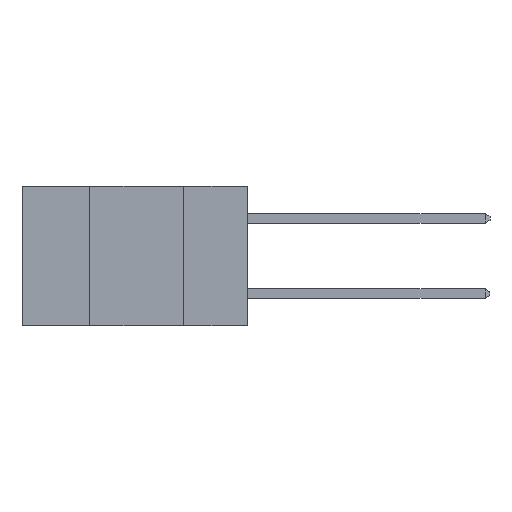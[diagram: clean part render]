
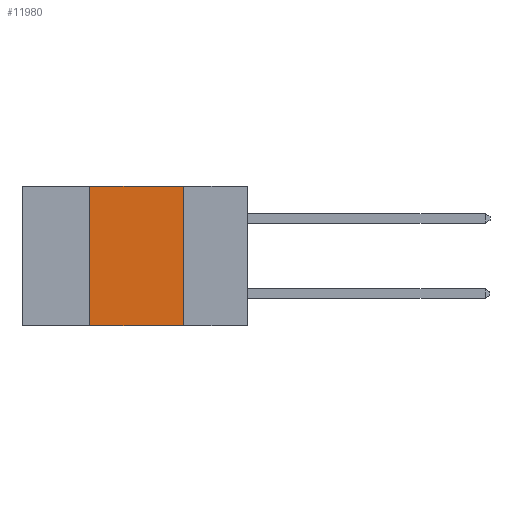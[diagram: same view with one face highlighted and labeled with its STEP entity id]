
A CAD part, left-side view. The second image highlights one B-rep face of the part: STEP entity #11980.
In plain terms, the highlighted planar face has unit normal (-1, 0, 0).
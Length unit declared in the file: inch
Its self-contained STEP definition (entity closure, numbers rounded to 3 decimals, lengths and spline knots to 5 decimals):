
#493 = VERTEX_POINT ( 'NONE', #1086 ) ;
#560 = VECTOR ( 'NONE', #1046, 39.37008 ) ;
#861 = ORIENTED_EDGE ( 'NONE', *, *, #2128, .F. ) ;
#951 = AXIS2_PLACEMENT_3D ( 'NONE', #5636, #13935, #6883 ) ;
#1046 = DIRECTION ( 'NONE',  ( 0., 0., -1. ) ) ;
#1086 = CARTESIAN_POINT ( 'NONE',  ( 0., 0.42, -0.37 ) ) ;
#1189 = CARTESIAN_POINT ( 'NONE',  ( 0., 0.42, 0. ) ) ;
#1529 = ORIENTED_EDGE ( 'NONE', *, *, #1826, .F. ) ;
#1552 = VECTOR ( 'NONE', #4815, 39.37008 ) ;
#1826 = EDGE_CURVE ( 'NONE', #493, #11767, #13750, .T. ) ;
#2088 = EDGE_LOOP ( 'NONE', ( #861, #12852, #1529, #9672 ) ) ;
#2112 = PLANE ( 'NONE',  #951 ) ;
#2128 = EDGE_CURVE ( 'NONE', #6800, #13142, #3761, .T. ) ;
#2711 = FACE_OUTER_BOUND ( 'NONE', #2088, .T. ) ;
#3250 = CARTESIAN_POINT ( 'NONE',  ( 0., 0.17, 0. ) ) ;
#3313 = CARTESIAN_POINT ( 'NONE',  ( 0., 0.6, 0. ) ) ;
#3456 = LINE ( 'NONE', #3313, #9105 ) ;
#3685 = EDGE_CURVE ( 'NONE', #493, #13142, #6511, .T. ) ;
#3761 = LINE ( 'NONE', #3250, #560 ) ;
#4409 = CARTESIAN_POINT ( 'NONE',  ( 0., 0.17, 0. ) ) ;
#4815 = DIRECTION ( 'NONE',  ( 0., 0., 1. ) ) ;
#5636 = CARTESIAN_POINT ( 'NONE',  ( 0., 0.6, 0. ) ) ;
#6507 = CARTESIAN_POINT ( 'NONE',  ( 0., 0.42, 0. ) ) ;
#6511 = LINE ( 'NONE', #13439, #9386 ) ;
#6800 = VERTEX_POINT ( 'NONE', #4409 ) ;
#6883 = DIRECTION ( 'NONE',  ( 0., 0., -1. ) ) ;
#7132 = DIRECTION ( 'NONE',  ( 0., -1., 0. ) ) ;
#7320 = EDGE_CURVE ( 'NONE', #11767, #6800, #3456, .T. ) ;
#9105 = VECTOR ( 'NONE', #7132, 39.37008 ) ;
#9386 = VECTOR ( 'NONE', #12937, 39.37008 ) ;
#9672 = ORIENTED_EDGE ( 'NONE', *, *, #3685, .T. ) ;
#11767 = VERTEX_POINT ( 'NONE', #6507 ) ;
#11980 = ADVANCED_FACE ( 'NONE', ( #2711 ), #2112, .F. ) ;
#12601 = CARTESIAN_POINT ( 'NONE',  ( 0., 0.17, -0.37 ) ) ;
#12852 = ORIENTED_EDGE ( 'NONE', *, *, #7320, .F. ) ;
#12937 = DIRECTION ( 'NONE',  ( 0., -1., 0. ) ) ;
#13142 = VERTEX_POINT ( 'NONE', #12601 ) ;
#13439 = CARTESIAN_POINT ( 'NONE',  ( 0., 0.6, -0.37 ) ) ;
#13750 = LINE ( 'NONE', #1189, #1552 ) ;
#13935 = DIRECTION ( 'NONE',  ( 1., 0., 0. ) ) ;
